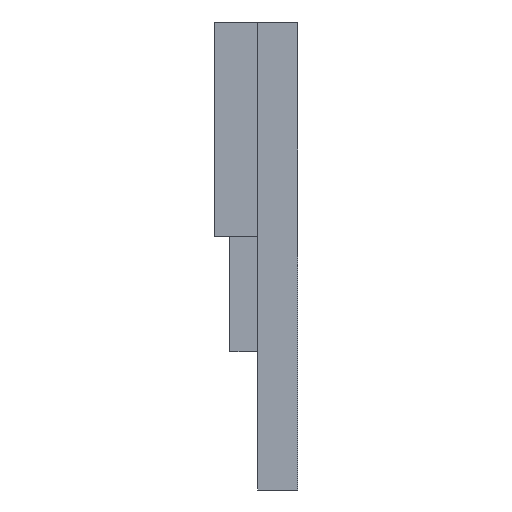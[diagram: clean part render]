
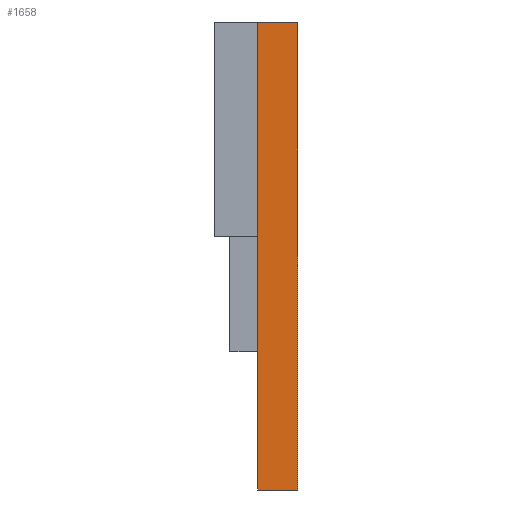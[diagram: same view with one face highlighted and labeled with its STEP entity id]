
A CAD part, left-side view. The second image highlights one B-rep face of the part: STEP entity #1658.
In plain terms, the highlighted planar face has unit normal (-1, 0, 0).
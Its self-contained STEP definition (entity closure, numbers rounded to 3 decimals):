
#25 = CARTESIAN_POINT ( 'NONE',  ( -93.25, 6.3, 36.5 ) ) ;
#87 = LINE ( 'NONE', #364, #703 ) ;
#117 = CARTESIAN_POINT ( 'NONE',  ( -93.25, 6.3, 36.5 ) ) ;
#125 = VECTOR ( 'NONE', #1205, 1000. ) ;
#133 = ORIENTED_EDGE ( 'NONE', *, *, #1296, .T. ) ;
#137 = DIRECTION ( 'NONE',  ( 1., 0., 0. ) ) ;
#187 = AXIS2_PLACEMENT_3D ( 'NONE', #117, #137, #1030 ) ;
#242 = EDGE_LOOP ( 'NONE', ( #1245, #1514, #652, #133 ) ) ;
#248 = VECTOR ( 'NONE', #522, 1000. ) ;
#290 = LINE ( 'NONE', #1111, #1398 ) ;
#317 = VERTEX_POINT ( 'NONE', #25 ) ;
#364 = CARTESIAN_POINT ( 'NONE',  ( -93.25, 6.3, 36.5 ) ) ;
#414 = EDGE_CURVE ( 'NONE', #1104, #317, #720, .T. ) ;
#522 = DIRECTION ( 'NONE',  ( 0., -1., 0. ) ) ;
#576 = DIRECTION ( 'NONE',  ( 0., 0., 1. ) ) ;
#652 = ORIENTED_EDGE ( 'NONE', *, *, #414, .F. ) ;
#681 = CARTESIAN_POINT ( 'NONE',  ( -93.25, 0., -36.5 ) ) ;
#703 = VECTOR ( 'NONE', #1124, 1000. ) ;
#720 = LINE ( 'NONE', #803, #125 ) ;
#754 = CARTESIAN_POINT ( 'NONE',  ( -93.25, 6.3, -36.5 ) ) ;
#803 = CARTESIAN_POINT ( 'NONE',  ( -93.25, 6.3, 36.5 ) ) ;
#908 = VERTEX_POINT ( 'NONE', #681 ) ;
#967 = CARTESIAN_POINT ( 'NONE',  ( -93.25, 6.3, -36.5 ) ) ;
#1030 = DIRECTION ( 'NONE',  ( 0., 0., -1. ) ) ;
#1039 = EDGE_CURVE ( 'NONE', #908, #1181, #290, .T. ) ;
#1104 = VERTEX_POINT ( 'NONE', #967 ) ;
#1111 = CARTESIAN_POINT ( 'NONE',  ( -93.25, 0., 36.5 ) ) ;
#1124 = DIRECTION ( 'NONE',  ( 0., -1., 0. ) ) ;
#1136 = CARTESIAN_POINT ( 'NONE',  ( -93.25, 0., 36.5 ) ) ;
#1171 = FACE_OUTER_BOUND ( 'NONE', #242, .T. ) ;
#1181 = VERTEX_POINT ( 'NONE', #1136 ) ;
#1205 = DIRECTION ( 'NONE',  ( 0., 0., 1. ) ) ;
#1245 = ORIENTED_EDGE ( 'NONE', *, *, #1039, .T. ) ;
#1296 = EDGE_CURVE ( 'NONE', #1104, #908, #1610, .T. ) ;
#1398 = VECTOR ( 'NONE', #576, 1000. ) ;
#1514 = ORIENTED_EDGE ( 'NONE', *, *, #1556, .F. ) ;
#1556 = EDGE_CURVE ( 'NONE', #317, #1181, #87, .T. ) ;
#1610 = LINE ( 'NONE', #754, #248 ) ;
#1645 = PLANE ( 'NONE',  #187 ) ;
#1658 = ADVANCED_FACE ( 'NONE', ( #1171 ), #1645, .F. ) ;
